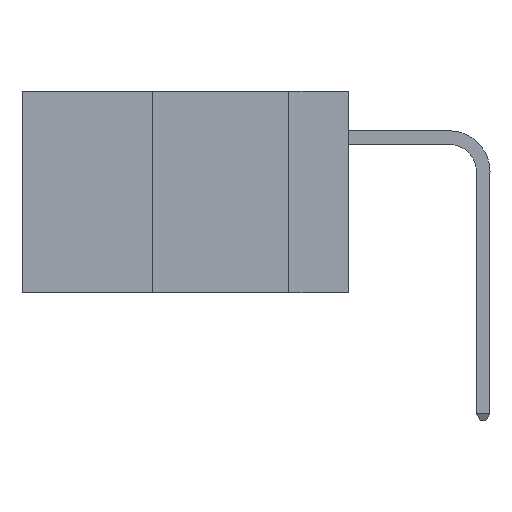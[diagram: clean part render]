
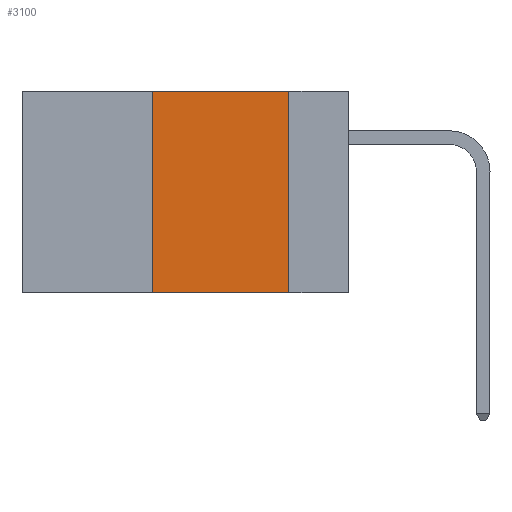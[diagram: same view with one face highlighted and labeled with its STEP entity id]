
A CAD part, left-side view. The second image highlights one B-rep face of the part: STEP entity #3100.
In plain terms, the highlighted planar face has unit normal (-1, 0, 0).
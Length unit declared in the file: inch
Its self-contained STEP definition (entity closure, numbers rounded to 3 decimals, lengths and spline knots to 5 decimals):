
#131 = EDGE_CURVE ( 'NONE', #7811, #8550, #14651, .T. ) ;
#646 = VECTOR ( 'NONE', #1583, 39.37008 ) ;
#903 = DIRECTION ( 'NONE',  ( 0., 0., 1. ) ) ;
#1179 = VERTEX_POINT ( 'NONE', #13073 ) ;
#1583 = DIRECTION ( 'NONE',  ( 0., -1., 0. ) ) ;
#1587 = CARTESIAN_POINT ( 'NONE',  ( 0., 0.11, -0.37 ) ) ;
#2377 = ORIENTED_EDGE ( 'NONE', *, *, #14315, .T. ) ;
#2561 = ORIENTED_EDGE ( 'NONE', *, *, #131, .F. ) ;
#3051 = CARTESIAN_POINT ( 'NONE',  ( 0., 0.6, 0. ) ) ;
#3100 = ADVANCED_FACE ( 'NONE', ( #14674 ), #10577, .F. ) ;
#4005 = LINE ( 'NONE', #10365, #646 ) ;
#4089 = CARTESIAN_POINT ( 'NONE',  ( 0., 0.11, 0. ) ) ;
#4621 = VECTOR ( 'NONE', #8616, 39.37008 ) ;
#4901 = ORIENTED_EDGE ( 'NONE', *, *, #7198, .F. ) ;
#5153 = CARTESIAN_POINT ( 'NONE',  ( 0., 0.11, 0. ) ) ;
#6784 = DIRECTION ( 'NONE',  ( 0., 0., -1. ) ) ;
#7198 = EDGE_CURVE ( 'NONE', #1179, #15872, #14824, .T. ) ;
#7811 = VERTEX_POINT ( 'NONE', #5153 ) ;
#8550 = VERTEX_POINT ( 'NONE', #1587 ) ;
#8616 = DIRECTION ( 'NONE',  ( 0., 0., -1. ) ) ;
#8755 = DIRECTION ( 'NONE',  ( 0., -1., 0. ) ) ;
#9472 = CARTESIAN_POINT ( 'NONE',  ( 0., 0.36, 0. ) ) ;
#9595 = AXIS2_PLACEMENT_3D ( 'NONE', #3051, #14389, #6784 ) ;
#10365 = CARTESIAN_POINT ( 'NONE',  ( 0., 0.6, 0. ) ) ;
#10577 = PLANE ( 'NONE',  #9595 ) ;
#11508 = VECTOR ( 'NONE', #903, 39.37008 ) ;
#12824 = LINE ( 'NONE', #14997, #15754 ) ;
#12995 = EDGE_CURVE ( 'NONE', #15872, #7811, #4005, .T. ) ;
#13073 = CARTESIAN_POINT ( 'NONE',  ( 0., 0.36, -0.37 ) ) ;
#14167 = ORIENTED_EDGE ( 'NONE', *, *, #12995, .F. ) ;
#14315 = EDGE_CURVE ( 'NONE', #1179, #8550, #12824, .T. ) ;
#14389 = DIRECTION ( 'NONE',  ( 1., 0., 0. ) ) ;
#14398 = EDGE_LOOP ( 'NONE', ( #2561, #14167, #4901, #2377 ) ) ;
#14651 = LINE ( 'NONE', #4089, #4621 ) ;
#14674 = FACE_OUTER_BOUND ( 'NONE', #14398, .T. ) ;
#14824 = LINE ( 'NONE', #15963, #11508 ) ;
#14997 = CARTESIAN_POINT ( 'NONE',  ( 0., 0.6, -0.37 ) ) ;
#15754 = VECTOR ( 'NONE', #8755, 39.37008 ) ;
#15872 = VERTEX_POINT ( 'NONE', #9472 ) ;
#15963 = CARTESIAN_POINT ( 'NONE',  ( 0., 0.36, 0. ) ) ;
